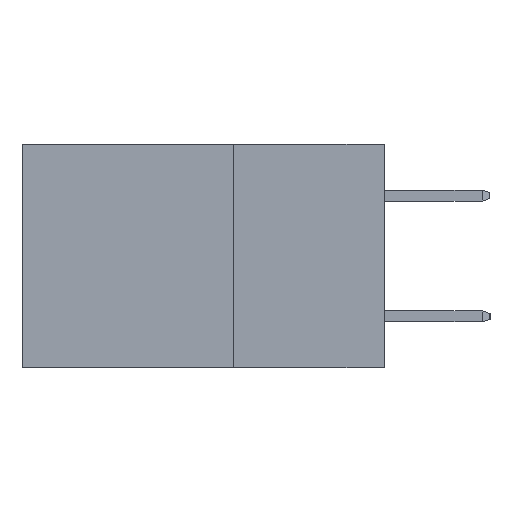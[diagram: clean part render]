
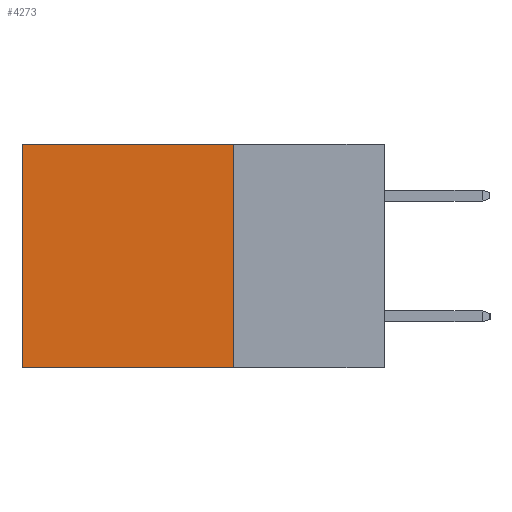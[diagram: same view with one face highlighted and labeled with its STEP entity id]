
A CAD part, left-side view. The second image highlights one B-rep face of the part: STEP entity #4273.
In plain terms, the highlighted planar face has unit normal (-1, 0, 0).
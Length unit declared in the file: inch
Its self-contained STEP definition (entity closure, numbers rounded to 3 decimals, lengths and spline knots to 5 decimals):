
#188 = ORIENTED_EDGE ( 'NONE', *, *, #3898, .T. ) ;
#576 = VECTOR ( 'NONE', #3697, 39.37008 ) ;
#1040 = LINE ( 'NONE', #3000, #576 ) ;
#1256 = VERTEX_POINT ( 'NONE', #4047 ) ;
#2036 = LINE ( 'NONE', #6241, #8790 ) ;
#2223 = EDGE_CURVE ( 'NONE', #3366, #6285, #1040, .T. ) ;
#2289 = VERTEX_POINT ( 'NONE', #3026 ) ;
#2503 = DIRECTION ( 'NONE',  ( 0., 0., -1. ) ) ;
#2526 = FACE_OUTER_BOUND ( 'NONE', #5424, .T. ) ;
#2652 = ORIENTED_EDGE ( 'NONE', *, *, #8586, .T. ) ;
#3000 = CARTESIAN_POINT ( 'NONE',  ( 0.2615, 0.25, -0.37 ) ) ;
#3026 = CARTESIAN_POINT ( 'NONE',  ( 0.2615, 0.6, 0. ) ) ;
#3366 = VERTEX_POINT ( 'NONE', #4892 ) ;
#3697 = DIRECTION ( 'NONE',  ( 0., 1., 0. ) ) ;
#3898 = EDGE_CURVE ( 'NONE', #2289, #6285, #4030, .T. ) ;
#4030 = LINE ( 'NONE', #7585, #6190 ) ;
#4047 = CARTESIAN_POINT ( 'NONE',  ( 0.2615, 0.25, 0. ) ) ;
#4273 = ADVANCED_FACE ( 'NONE', ( #2526 ), #6205, .F. ) ;
#4292 = ORIENTED_EDGE ( 'NONE', *, *, #2223, .F. ) ;
#4892 = CARTESIAN_POINT ( 'NONE',  ( 0.2615, 0.25, -0.37 ) ) ;
#4917 = CARTESIAN_POINT ( 'NONE',  ( 0.2615, 0.25, 0. ) ) ;
#4993 = EDGE_CURVE ( 'NONE', #1256, #3366, #2036, .T. ) ;
#5121 = AXIS2_PLACEMENT_3D ( 'NONE', #6489, #6073, #6071 ) ;
#5424 = EDGE_LOOP ( 'NONE', ( #188, #4292, #7872, #2652 ) ) ;
#5517 = CARTESIAN_POINT ( 'NONE',  ( 0.2615, 0.6, -0.37 ) ) ;
#5601 = DIRECTION ( 'NONE',  ( 0., 1., 0. ) ) ;
#6071 = DIRECTION ( 'NONE',  ( 0., 0., -1. ) ) ;
#6073 = DIRECTION ( 'NONE',  ( 1., 0., 0. ) ) ;
#6190 = VECTOR ( 'NONE', #7582, 39.37008 ) ;
#6205 = PLANE ( 'NONE',  #5121 ) ;
#6241 = CARTESIAN_POINT ( 'NONE',  ( 0.2615, 0.25, -0.37 ) ) ;
#6285 = VERTEX_POINT ( 'NONE', #5517 ) ;
#6489 = CARTESIAN_POINT ( 'NONE',  ( 0.2615, 0.25, -0.37 ) ) ;
#7582 = DIRECTION ( 'NONE',  ( 0., 0., -1. ) ) ;
#7585 = CARTESIAN_POINT ( 'NONE',  ( 0.2615, 0.6, -0.37 ) ) ;
#7872 = ORIENTED_EDGE ( 'NONE', *, *, #4993, .F. ) ;
#8423 = VECTOR ( 'NONE', #5601, 39.37008 ) ;
#8586 = EDGE_CURVE ( 'NONE', #1256, #2289, #8617, .T. ) ;
#8617 = LINE ( 'NONE', #4917, #8423 ) ;
#8790 = VECTOR ( 'NONE', #2503, 39.37008 ) ;
